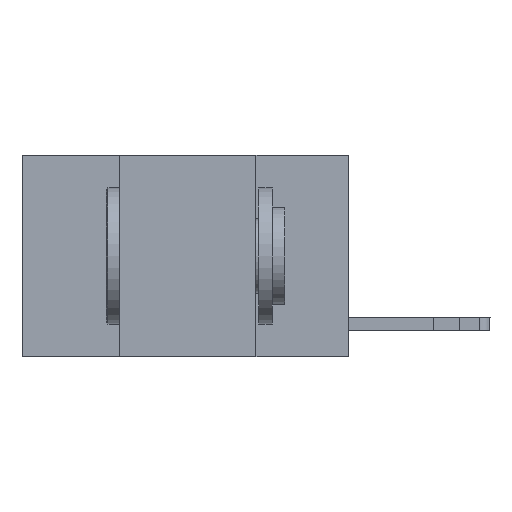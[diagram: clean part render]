
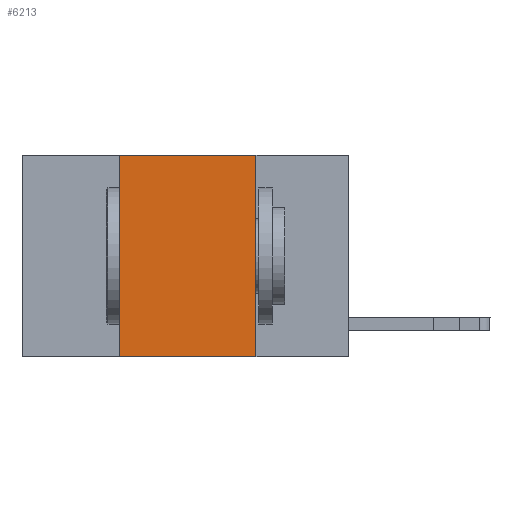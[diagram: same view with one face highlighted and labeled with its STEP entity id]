
A CAD part, left-side view. The second image highlights one B-rep face of the part: STEP entity #6213.
In plain terms, the highlighted planar face has unit normal (-1, 0, 0).
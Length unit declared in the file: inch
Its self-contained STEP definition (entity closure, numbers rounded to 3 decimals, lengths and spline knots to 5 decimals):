
#784 = ORIENTED_EDGE ( 'NONE', *, *, #12012, .F. ) ;
#984 = EDGE_CURVE ( 'NONE', #12164, #14358, #5970, .T. ) ;
#1183 = CARTESIAN_POINT ( 'NONE',  ( 0., 0.42, -0.37 ) ) ;
#1188 = PLANE ( 'NONE',  #4873 ) ;
#1389 = LINE ( 'NONE', #13951, #10542 ) ;
#2091 = CARTESIAN_POINT ( 'NONE',  ( 0., 0.42, 0. ) ) ;
#3314 = LINE ( 'NONE', #7813, #9585 ) ;
#4403 = LINE ( 'NONE', #11130, #13413 ) ;
#4580 = DIRECTION ( 'NONE',  ( 0., 0., -1. ) ) ;
#4669 = ORIENTED_EDGE ( 'NONE', *, *, #10020, .T. ) ;
#4873 = AXIS2_PLACEMENT_3D ( 'NONE', #11446, #10196, #4580 ) ;
#5013 = DIRECTION ( 'NONE',  ( 0., 0., -1. ) ) ;
#5970 = LINE ( 'NONE', #8416, #9037 ) ;
#6213 = ADVANCED_FACE ( 'NONE', ( #6779 ), #1188, .F. ) ;
#6702 = DIRECTION ( 'NONE',  ( 0., -1., 0. ) ) ;
#6779 = FACE_OUTER_BOUND ( 'NONE', #11702, .T. ) ;
#7813 = CARTESIAN_POINT ( 'NONE',  ( 0., 0.6, -0.37 ) ) ;
#7922 = DIRECTION ( 'NONE',  ( 0., 0., 1. ) ) ;
#8416 = CARTESIAN_POINT ( 'NONE',  ( 0., 0.17, 0. ) ) ;
#9037 = VECTOR ( 'NONE', #5013, 39.37008 ) ;
#9224 = ORIENTED_EDGE ( 'NONE', *, *, #10129, .F. ) ;
#9474 = VERTEX_POINT ( 'NONE', #2091 ) ;
#9585 = VECTOR ( 'NONE', #6702, 39.37008 ) ;
#10020 = EDGE_CURVE ( 'NONE', #10061, #14358, #3314, .T. ) ;
#10061 = VERTEX_POINT ( 'NONE', #1183 ) ;
#10129 = EDGE_CURVE ( 'NONE', #9474, #12164, #1389, .T. ) ;
#10196 = DIRECTION ( 'NONE',  ( 1., 0., 0. ) ) ;
#10220 = CARTESIAN_POINT ( 'NONE',  ( 0., 0.17, -0.37 ) ) ;
#10542 = VECTOR ( 'NONE', #12632, 39.37008 ) ;
#11130 = CARTESIAN_POINT ( 'NONE',  ( 0., 0.42, 0. ) ) ;
#11446 = CARTESIAN_POINT ( 'NONE',  ( 0., 0.6, 0. ) ) ;
#11635 = CARTESIAN_POINT ( 'NONE',  ( 0., 0.17, 0. ) ) ;
#11702 = EDGE_LOOP ( 'NONE', ( #14439, #9224, #784, #4669 ) ) ;
#12012 = EDGE_CURVE ( 'NONE', #10061, #9474, #4403, .T. ) ;
#12164 = VERTEX_POINT ( 'NONE', #11635 ) ;
#12632 = DIRECTION ( 'NONE',  ( 0., -1., 0. ) ) ;
#13413 = VECTOR ( 'NONE', #7922, 39.37008 ) ;
#13951 = CARTESIAN_POINT ( 'NONE',  ( 0., 0.6, 0. ) ) ;
#14358 = VERTEX_POINT ( 'NONE', #10220 ) ;
#14439 = ORIENTED_EDGE ( 'NONE', *, *, #984, .F. ) ;
